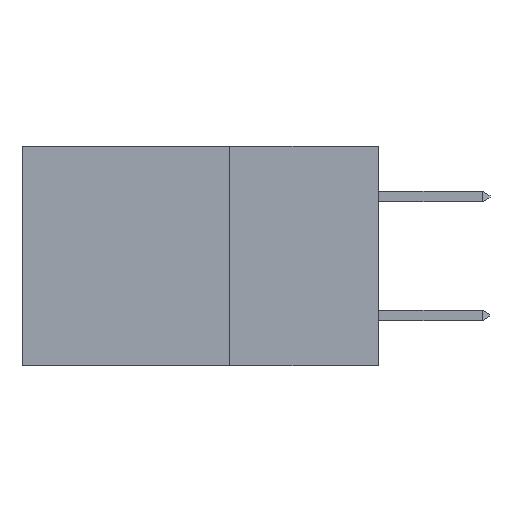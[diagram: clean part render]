
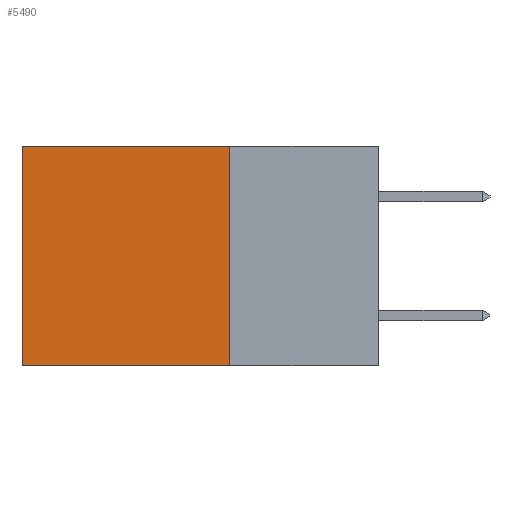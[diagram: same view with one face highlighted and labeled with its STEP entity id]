
A CAD part, left-side view. The second image highlights one B-rep face of the part: STEP entity #5490.
In plain terms, the highlighted planar face has unit normal (-1, 0, 0).
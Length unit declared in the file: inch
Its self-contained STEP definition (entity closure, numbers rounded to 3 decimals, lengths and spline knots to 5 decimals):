
#53 = VECTOR ( 'NONE', #9042, 39.37008 ) ;
#784 = VECTOR ( 'NONE', #10063, 39.37008 ) ;
#1103 = LINE ( 'NONE', #5036, #784 ) ;
#1643 = EDGE_CURVE ( 'NONE', #2005, #5928, #5176, .T. ) ;
#1991 = VERTEX_POINT ( 'NONE', #4505 ) ;
#2005 = VERTEX_POINT ( 'NONE', #6052 ) ;
#2306 = PLANE ( 'NONE',  #2696 ) ;
#2696 = AXIS2_PLACEMENT_3D ( 'NONE', #2992, #6314, #7109 ) ;
#2992 = CARTESIAN_POINT ( 'NONE',  ( 0.298, 0.25, 0. ) ) ;
#3042 = CARTESIAN_POINT ( 'NONE',  ( 0.298, 0.6, -0.37 ) ) ;
#3091 = EDGE_CURVE ( 'NONE', #1991, #9584, #7465, .T. ) ;
#4505 = CARTESIAN_POINT ( 'NONE',  ( 0.298, 0.25, 0. ) ) ;
#4844 = VECTOR ( 'NONE', #7432, 39.37008 ) ;
#4845 = CARTESIAN_POINT ( 'NONE',  ( 0.298, 0.25, -0.37 ) ) ;
#5036 = CARTESIAN_POINT ( 'NONE',  ( 0.298, 0.25, 0. ) ) ;
#5098 = CARTESIAN_POINT ( 'NONE',  ( 0.298, 0.25, -0.37 ) ) ;
#5176 = LINE ( 'NONE', #8893, #53 ) ;
#5490 = ADVANCED_FACE ( 'NONE', ( #8834 ), #2306, .F. ) ;
#5928 = VERTEX_POINT ( 'NONE', #3042 ) ;
#6052 = CARTESIAN_POINT ( 'NONE',  ( 0.298, 0.6, 0. ) ) ;
#6314 = DIRECTION ( 'NONE',  ( 1., 0., 0. ) ) ;
#7109 = DIRECTION ( 'NONE',  ( 0., 0., -1. ) ) ;
#7432 = DIRECTION ( 'NONE',  ( 0., 0., -1. ) ) ;
#7465 = LINE ( 'NONE', #7641, #4844 ) ;
#7641 = CARTESIAN_POINT ( 'NONE',  ( 0.298, 0.25, 0. ) ) ;
#7824 = EDGE_LOOP ( 'NONE', ( #9101, #9444, #10460, #9466 ) ) ;
#7853 = EDGE_CURVE ( 'NONE', #9584, #5928, #9342, .T. ) ;
#8027 = EDGE_CURVE ( 'NONE', #1991, #2005, #1103, .T. ) ;
#8834 = FACE_OUTER_BOUND ( 'NONE', #7824, .T. ) ;
#8893 = CARTESIAN_POINT ( 'NONE',  ( 0.298, 0.6, 0. ) ) ;
#9042 = DIRECTION ( 'NONE',  ( 0., 0., -1. ) ) ;
#9101 = ORIENTED_EDGE ( 'NONE', *, *, #1643, .T. ) ;
#9342 = LINE ( 'NONE', #4845, #11170 ) ;
#9444 = ORIENTED_EDGE ( 'NONE', *, *, #7853, .F. ) ;
#9466 = ORIENTED_EDGE ( 'NONE', *, *, #8027, .T. ) ;
#9584 = VERTEX_POINT ( 'NONE', #5098 ) ;
#10063 = DIRECTION ( 'NONE',  ( 0., 1., 0. ) ) ;
#10460 = ORIENTED_EDGE ( 'NONE', *, *, #3091, .F. ) ;
#10721 = DIRECTION ( 'NONE',  ( 0., 1., 0. ) ) ;
#11170 = VECTOR ( 'NONE', #10721, 39.37008 ) ;
